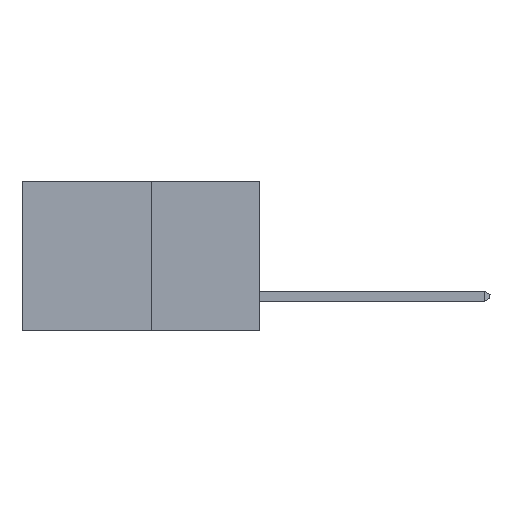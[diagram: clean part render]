
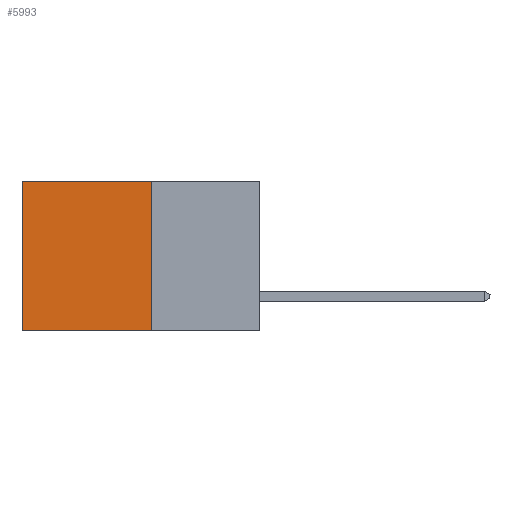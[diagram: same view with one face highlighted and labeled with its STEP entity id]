
A CAD part, left-side view. The second image highlights one B-rep face of the part: STEP entity #5993.
In plain terms, the highlighted planar face has unit normal (-1, 0, 0).
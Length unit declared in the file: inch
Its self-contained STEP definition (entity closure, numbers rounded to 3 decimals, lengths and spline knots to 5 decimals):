
#825 = EDGE_LOOP ( 'NONE', ( #5315, #7807, #5240, #8954 ) ) ;
#1276 = VECTOR ( 'NONE', #4425, 39.37008 ) ;
#1490 = VECTOR ( 'NONE', #4393, 39.37008 ) ;
#1590 = CARTESIAN_POINT ( 'NONE',  ( 0.277, 0.59, -0.37 ) ) ;
#1797 = LINE ( 'NONE', #7858, #1490 ) ;
#2228 = VECTOR ( 'NONE', #5941, 39.37008 ) ;
#4002 = FACE_OUTER_BOUND ( 'NONE', #825, .T. ) ;
#4165 = EDGE_CURVE ( 'NONE', #4846, #6885, #1797, .T. ) ;
#4393 = DIRECTION ( 'NONE',  ( 0., 0., -1. ) ) ;
#4425 = DIRECTION ( 'NONE',  ( 0., 0., -1. ) ) ;
#4592 = CARTESIAN_POINT ( 'NONE',  ( 0.277, 0.59, -0.37 ) ) ;
#4846 = VERTEX_POINT ( 'NONE', #9777 ) ;
#5240 = ORIENTED_EDGE ( 'NONE', *, *, #4165, .F. ) ;
#5286 = VECTOR ( 'NONE', #10943, 39.37008 ) ;
#5301 = LINE ( 'NONE', #5875, #2228 ) ;
#5315 = ORIENTED_EDGE ( 'NONE', *, *, #6251, .T. ) ;
#5695 = CARTESIAN_POINT ( 'NONE',  ( 0.277, 0.27, -0.37 ) ) ;
#5875 = CARTESIAN_POINT ( 'NONE',  ( 0.277, 0.27, 0. ) ) ;
#5941 = DIRECTION ( 'NONE',  ( 0., 1., 0. ) ) ;
#5993 = ADVANCED_FACE ( 'NONE', ( #4002 ), #8290, .F. ) ;
#6251 = EDGE_CURVE ( 'NONE', #7826, #11691, #12420, .T. ) ;
#6885 = VERTEX_POINT ( 'NONE', #11568 ) ;
#7807 = ORIENTED_EDGE ( 'NONE', *, *, #8815, .F. ) ;
#7826 = VERTEX_POINT ( 'NONE', #10044 ) ;
#7858 = CARTESIAN_POINT ( 'NONE',  ( 0.277, 0.27, -0.37 ) ) ;
#8033 = EDGE_CURVE ( 'NONE', #4846, #7826, #5301, .T. ) ;
#8197 = DIRECTION ( 'NONE',  ( 0., 0., -1. ) ) ;
#8235 = LINE ( 'NONE', #5695, #5286 ) ;
#8255 = DIRECTION ( 'NONE',  ( 1., 0., 0. ) ) ;
#8271 = CARTESIAN_POINT ( 'NONE',  ( 0.277, 0.27, -0.37 ) ) ;
#8290 = PLANE ( 'NONE',  #8618 ) ;
#8618 = AXIS2_PLACEMENT_3D ( 'NONE', #8271, #8255, #8197 ) ;
#8815 = EDGE_CURVE ( 'NONE', #6885, #11691, #8235, .T. ) ;
#8954 = ORIENTED_EDGE ( 'NONE', *, *, #8033, .T. ) ;
#9777 = CARTESIAN_POINT ( 'NONE',  ( 0.277, 0.27, 0. ) ) ;
#10044 = CARTESIAN_POINT ( 'NONE',  ( 0.277, 0.59, 0. ) ) ;
#10943 = DIRECTION ( 'NONE',  ( 0., 1., 0. ) ) ;
#11568 = CARTESIAN_POINT ( 'NONE',  ( 0.277, 0.27, -0.37 ) ) ;
#11691 = VERTEX_POINT ( 'NONE', #1590 ) ;
#12420 = LINE ( 'NONE', #4592, #1276 ) ;
